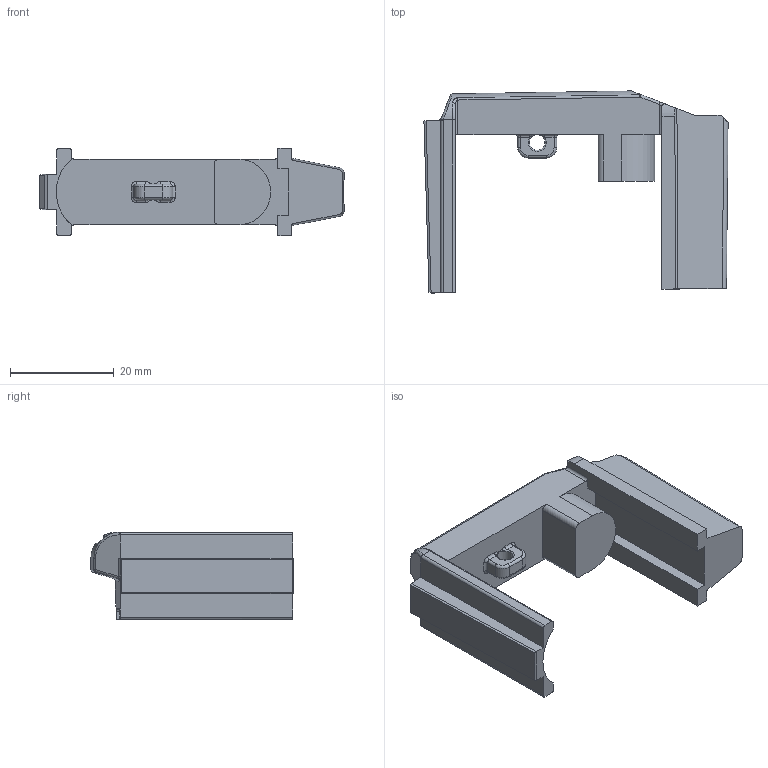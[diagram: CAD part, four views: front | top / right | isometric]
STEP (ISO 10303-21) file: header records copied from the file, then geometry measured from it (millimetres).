
FILE_DESCRIPTION(('FreeCAD Model'),'2;1');
FILE_NAME('Open CASCADE Shape Model','2025-07-16T20:18:11',(''),(''), 'Open CASCADE STEP processor 7.8','FreeCAD','Unknown');
FILE_SCHEMA(('AUTOMOTIVE_DESIGN { 1 0 10303 214 1 1 1 1 }'));
Length unit declared in the file: millimetre
Products named in the file (1): Cut002
Bounding box: 58.53 x 38.89 x 16.85 mm (x, y, z)
Volume: 9832.4 mm3; surface area: 5892.8 mm2
Topology: 1 solids, 1 shells, 138 faces, 367 edges, 220 vertices
Faces by surface type: cylinder 46, plane 44, bspline 30, torus 14, sphere 4
Full cylindrical faces by diameter (mm): 3 x1
Entity records: 5173 total; most frequent: CARTESIAN_POINT 2046, ORIENTED_EDGE 714, DIRECTION 584, EDGE_CURVE 357, VERTEX_POINT 220, AXIS2_PLACEMENT_3D 209, LINE 166, VECTOR 166
